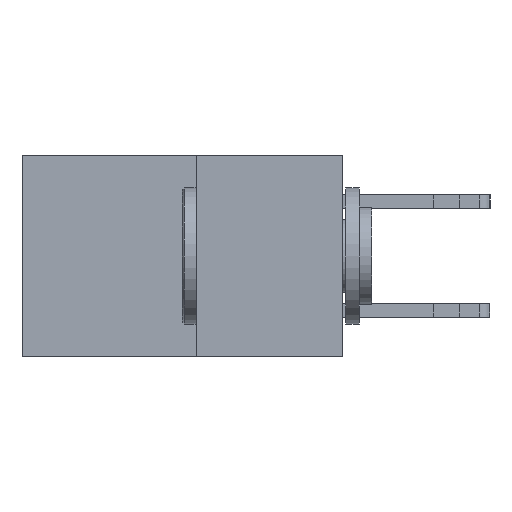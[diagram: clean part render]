
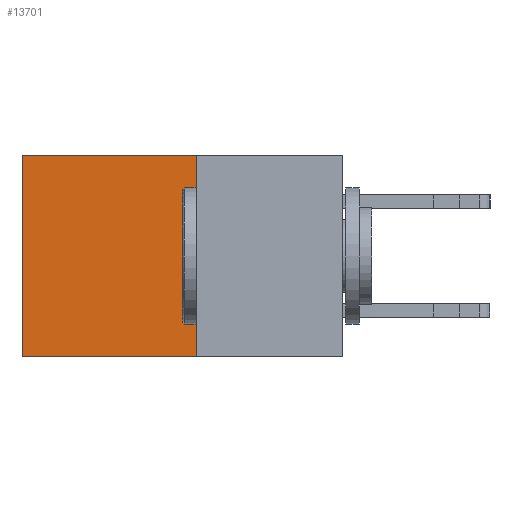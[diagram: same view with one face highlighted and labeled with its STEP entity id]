
A CAD part, left-side view. The second image highlights one B-rep face of the part: STEP entity #13701.
In plain terms, the highlighted planar face has unit normal (-1, 0, 0).
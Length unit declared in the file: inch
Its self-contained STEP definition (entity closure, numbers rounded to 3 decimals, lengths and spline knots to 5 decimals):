
#391 = ORIENTED_EDGE ( 'NONE', *, *, #23976, .T. ) ;
#612 = EDGE_CURVE ( 'NONE', #6327, #11092, #7370, .T. ) ;
#1040 = LINE ( 'NONE', #1165, #12645 ) ;
#1165 = CARTESIAN_POINT ( 'NONE',  ( 0.277, 0.27, 0. ) ) ;
#1960 = FACE_OUTER_BOUND ( 'NONE', #6349, .T. ) ;
#2553 = DIRECTION ( 'NONE',  ( 1., 0., 0. ) ) ;
#5596 = EDGE_CURVE ( 'NONE', #14280, #11092, #19629, .T. ) ;
#6123 = ORIENTED_EDGE ( 'NONE', *, *, #5596, .F. ) ;
#6327 = VERTEX_POINT ( 'NONE', #6608 ) ;
#6349 = EDGE_LOOP ( 'NONE', ( #9273, #6123, #24229, #391 ) ) ;
#6608 = CARTESIAN_POINT ( 'NONE',  ( 0.277, 0.59, 0. ) ) ;
#7370 = LINE ( 'NONE', #30048, #19070 ) ;
#9273 = ORIENTED_EDGE ( 'NONE', *, *, #612, .T. ) ;
#9584 = DIRECTION ( 'NONE',  ( 0., 0., -1. ) ) ;
#11092 = VERTEX_POINT ( 'NONE', #15839 ) ;
#11121 = VERTEX_POINT ( 'NONE', #15501 ) ;
#11545 = VECTOR ( 'NONE', #14734, 39.37008 ) ;
#11827 = VECTOR ( 'NONE', #9584, 39.37008 ) ;
#12645 = VECTOR ( 'NONE', #15059, 39.37008 ) ;
#13596 = CARTESIAN_POINT ( 'NONE',  ( 0.277, 0.27, -0.37 ) ) ;
#13701 = ADVANCED_FACE ( 'NONE', ( #1960 ), #14100, .F. ) ;
#14100 = PLANE ( 'NONE',  #20911 ) ;
#14280 = VERTEX_POINT ( 'NONE', #16026 ) ;
#14734 = DIRECTION ( 'NONE',  ( 0., 1., 0. ) ) ;
#15059 = DIRECTION ( 'NONE',  ( 0., 1., 0. ) ) ;
#15501 = CARTESIAN_POINT ( 'NONE',  ( 0.277, 0.27, 0. ) ) ;
#15839 = CARTESIAN_POINT ( 'NONE',  ( 0.277, 0.59, -0.37 ) ) ;
#16026 = CARTESIAN_POINT ( 'NONE',  ( 0.277, 0.27, -0.37 ) ) ;
#16464 = CARTESIAN_POINT ( 'NONE',  ( 0.277, 0.27, -0.37 ) ) ;
#18067 = LINE ( 'NONE', #25925, #11827 ) ;
#18830 = DIRECTION ( 'NONE',  ( 0., 0., -1. ) ) ;
#19070 = VECTOR ( 'NONE', #24249, 39.37008 ) ;
#19629 = LINE ( 'NONE', #13596, #11545 ) ;
#20911 = AXIS2_PLACEMENT_3D ( 'NONE', #16464, #2553, #18830 ) ;
#21109 = EDGE_CURVE ( 'NONE', #11121, #14280, #18067, .T. ) ;
#23976 = EDGE_CURVE ( 'NONE', #11121, #6327, #1040, .T. ) ;
#24229 = ORIENTED_EDGE ( 'NONE', *, *, #21109, .F. ) ;
#24249 = DIRECTION ( 'NONE',  ( 0., 0., -1. ) ) ;
#25925 = CARTESIAN_POINT ( 'NONE',  ( 0.277, 0.27, -0.37 ) ) ;
#30048 = CARTESIAN_POINT ( 'NONE',  ( 0.277, 0.59, -0.37 ) ) ;
